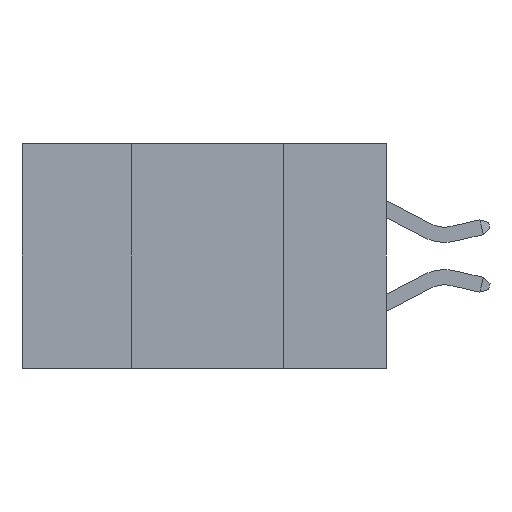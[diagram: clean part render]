
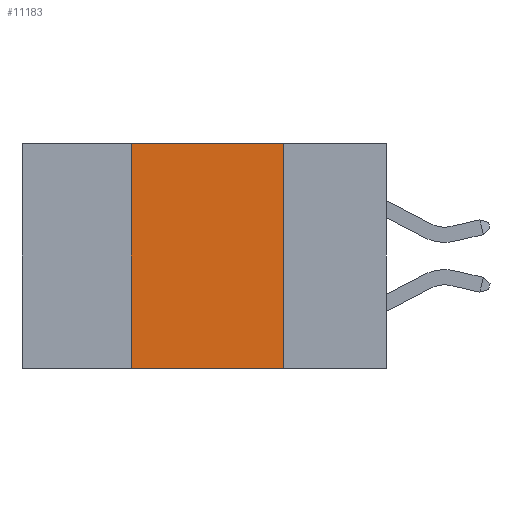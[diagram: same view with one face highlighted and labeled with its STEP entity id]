
A CAD part, left-side view. The second image highlights one B-rep face of the part: STEP entity #11183.
In plain terms, the highlighted planar face has unit normal (-1, 0, 0).
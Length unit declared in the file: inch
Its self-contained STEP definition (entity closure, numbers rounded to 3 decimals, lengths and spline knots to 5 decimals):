
#274 = DIRECTION ( 'NONE',  ( 0., 0., 1. ) ) ;
#843 = ORIENTED_EDGE ( 'NONE', *, *, #23868, .F. ) ;
#1480 = ORIENTED_EDGE ( 'NONE', *, *, #25666, .F. ) ;
#2066 = DIRECTION ( 'NONE',  ( 0., -1., 0. ) ) ;
#3259 = LINE ( 'NONE', #24359, #7941 ) ;
#3508 = CARTESIAN_POINT ( 'NONE',  ( 0., 0.17, -0.37 ) ) ;
#4356 = VERTEX_POINT ( 'NONE', #3508 ) ;
#4971 = VERTEX_POINT ( 'NONE', #19532 ) ;
#6532 = DIRECTION ( 'NONE',  ( 0., 0., -1. ) ) ;
#7045 = LINE ( 'NONE', #15975, #17616 ) ;
#7340 = LINE ( 'NONE', #18646, #23151 ) ;
#7941 = VECTOR ( 'NONE', #6532, 39.37008 ) ;
#8496 = DIRECTION ( 'NONE',  ( 0., 0., -1. ) ) ;
#8660 = FACE_OUTER_BOUND ( 'NONE', #17181, .T. ) ;
#8764 = DIRECTION ( 'NONE',  ( 0., -1., 0. ) ) ;
#11183 = ADVANCED_FACE ( 'NONE', ( #8660 ), #16408, .F. ) ;
#12804 = EDGE_CURVE ( 'NONE', #18298, #4356, #3259, .T. ) ;
#13951 = CARTESIAN_POINT ( 'NONE',  ( 0., 0.42, -0.37 ) ) ;
#15975 = CARTESIAN_POINT ( 'NONE',  ( 0., 0.6, 0. ) ) ;
#16408 = PLANE ( 'NONE',  #16457 ) ;
#16457 = AXIS2_PLACEMENT_3D ( 'NONE', #18369, #20369, #8496 ) ;
#16554 = VERTEX_POINT ( 'NONE', #13951 ) ;
#17181 = EDGE_LOOP ( 'NONE', ( #17926, #1480, #843, #23581 ) ) ;
#17616 = VECTOR ( 'NONE', #2066, 39.37008 ) ;
#17926 = ORIENTED_EDGE ( 'NONE', *, *, #12804, .F. ) ;
#18298 = VERTEX_POINT ( 'NONE', #19633 ) ;
#18369 = CARTESIAN_POINT ( 'NONE',  ( 0., 0.6, 0. ) ) ;
#18646 = CARTESIAN_POINT ( 'NONE',  ( 0., 0.6, -0.37 ) ) ;
#19532 = CARTESIAN_POINT ( 'NONE',  ( 0., 0.42, 0. ) ) ;
#19633 = CARTESIAN_POINT ( 'NONE',  ( 0., 0.17, 0. ) ) ;
#20369 = DIRECTION ( 'NONE',  ( 1., 0., 0. ) ) ;
#21694 = VECTOR ( 'NONE', #274, 39.37008 ) ;
#22919 = LINE ( 'NONE', #23979, #21694 ) ;
#23151 = VECTOR ( 'NONE', #8764, 39.37008 ) ;
#23581 = ORIENTED_EDGE ( 'NONE', *, *, #25213, .T. ) ;
#23868 = EDGE_CURVE ( 'NONE', #16554, #4971, #22919, .T. ) ;
#23979 = CARTESIAN_POINT ( 'NONE',  ( 0., 0.42, -0.37 ) ) ;
#24359 = CARTESIAN_POINT ( 'NONE',  ( 0., 0.17, -0.37 ) ) ;
#25213 = EDGE_CURVE ( 'NONE', #16554, #4356, #7340, .T. ) ;
#25666 = EDGE_CURVE ( 'NONE', #4971, #18298, #7045, .T. ) ;
